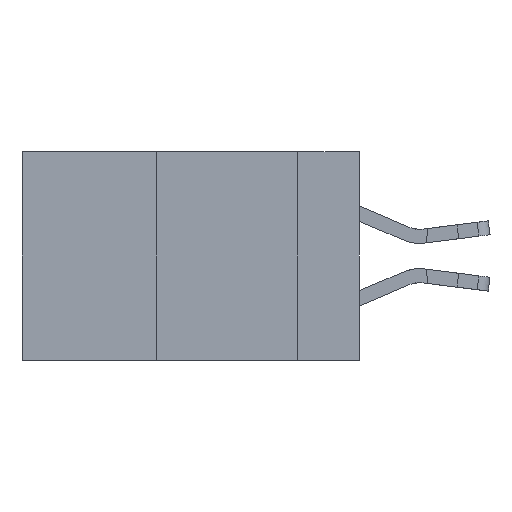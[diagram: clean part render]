
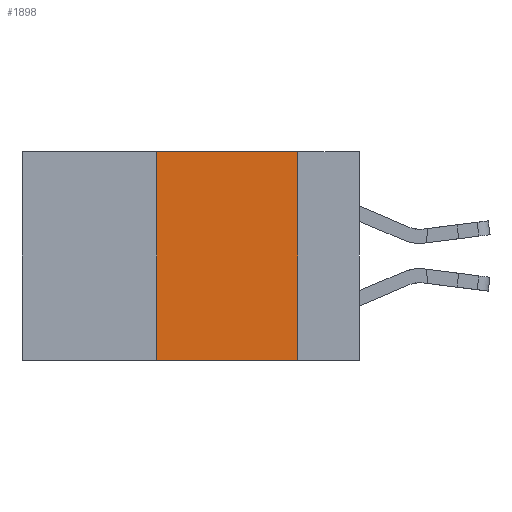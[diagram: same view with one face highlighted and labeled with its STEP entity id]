
A CAD part, left-side view. The second image highlights one B-rep face of the part: STEP entity #1898.
In plain terms, the highlighted planar face has unit normal (-1, 0, 0).
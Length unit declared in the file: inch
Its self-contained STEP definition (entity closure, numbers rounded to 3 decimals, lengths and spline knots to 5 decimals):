
#393 = CARTESIAN_POINT ( 'NONE',  ( 0., 0.11, 0. ) ) ;
#470 = LINE ( 'NONE', #3213, #16441 ) ;
#557 = DIRECTION ( 'NONE',  ( 1., 0., 0. ) ) ;
#786 = AXIS2_PLACEMENT_3D ( 'NONE', #12865, #557, #16988 ) ;
#1137 = CARTESIAN_POINT ( 'NONE',  ( 0., 0.11, 0. ) ) ;
#1898 = ADVANCED_FACE ( 'NONE', ( #2281 ), #7570, .F. ) ;
#2281 = FACE_OUTER_BOUND ( 'NONE', #13985, .T. ) ;
#2521 = LINE ( 'NONE', #6077, #9313 ) ;
#2781 = DIRECTION ( 'NONE',  ( 0., 0., 1. ) ) ;
#3079 = LINE ( 'NONE', #12984, #9803 ) ;
#3213 = CARTESIAN_POINT ( 'NONE',  ( 0., 0.36, 0. ) ) ;
#4478 = VECTOR ( 'NONE', #7337, 39.37008 ) ;
#4600 = ORIENTED_EDGE ( 'NONE', *, *, #11758, .F. ) ;
#4881 = LINE ( 'NONE', #393, #4478 ) ;
#6077 = CARTESIAN_POINT ( 'NONE',  ( 0., 0.6, -0.37 ) ) ;
#6114 = EDGE_CURVE ( 'NONE', #9838, #7060, #470, .T. ) ;
#6619 = EDGE_CURVE ( 'NONE', #10070, #10612, #4881, .T. ) ;
#7060 = VERTEX_POINT ( 'NONE', #13469 ) ;
#7337 = DIRECTION ( 'NONE',  ( 0., 0., -1. ) ) ;
#7427 = DIRECTION ( 'NONE',  ( 0., -1., 0. ) ) ;
#7570 = PLANE ( 'NONE',  #786 ) ;
#8845 = CARTESIAN_POINT ( 'NONE',  ( 0., 0.36, -0.37 ) ) ;
#9271 = ORIENTED_EDGE ( 'NONE', *, *, #14614, .T. ) ;
#9313 = VECTOR ( 'NONE', #7427, 39.37008 ) ;
#9803 = VECTOR ( 'NONE', #13037, 39.37008 ) ;
#9838 = VERTEX_POINT ( 'NONE', #8845 ) ;
#10070 = VERTEX_POINT ( 'NONE', #1137 ) ;
#10388 = ORIENTED_EDGE ( 'NONE', *, *, #6619, .F. ) ;
#10612 = VERTEX_POINT ( 'NONE', #16822 ) ;
#11758 = EDGE_CURVE ( 'NONE', #7060, #10070, #3079, .T. ) ;
#12865 = CARTESIAN_POINT ( 'NONE',  ( 0., 0.6, 0. ) ) ;
#12984 = CARTESIAN_POINT ( 'NONE',  ( 0., 0.6, 0. ) ) ;
#13037 = DIRECTION ( 'NONE',  ( 0., -1., 0. ) ) ;
#13469 = CARTESIAN_POINT ( 'NONE',  ( 0., 0.36, 0. ) ) ;
#13985 = EDGE_LOOP ( 'NONE', ( #10388, #4600, #15193, #9271 ) ) ;
#14614 = EDGE_CURVE ( 'NONE', #9838, #10612, #2521, .T. ) ;
#15193 = ORIENTED_EDGE ( 'NONE', *, *, #6114, .F. ) ;
#16441 = VECTOR ( 'NONE', #2781, 39.37008 ) ;
#16822 = CARTESIAN_POINT ( 'NONE',  ( 0., 0.11, -0.37 ) ) ;
#16988 = DIRECTION ( 'NONE',  ( 0., 0., -1. ) ) ;
